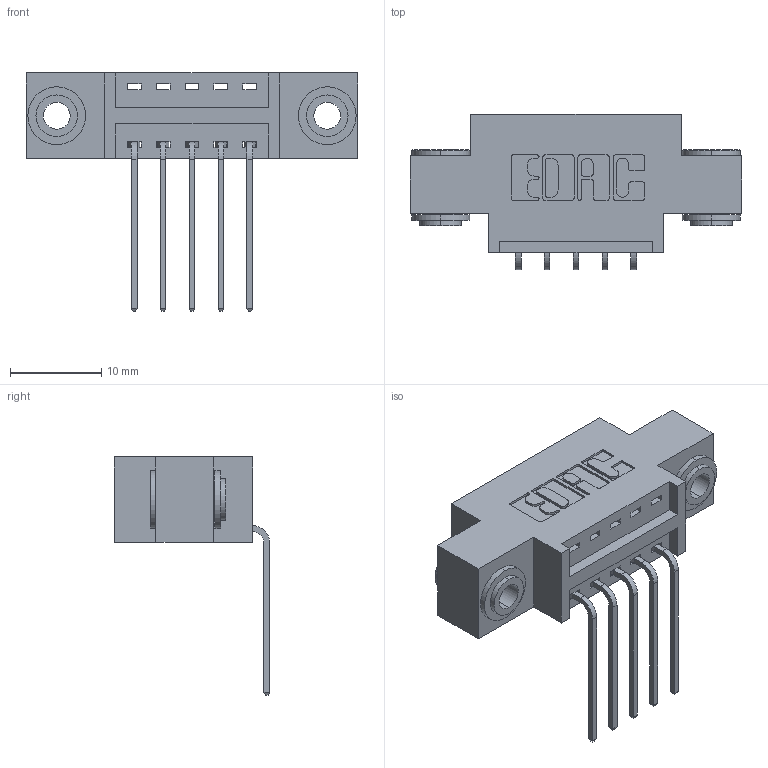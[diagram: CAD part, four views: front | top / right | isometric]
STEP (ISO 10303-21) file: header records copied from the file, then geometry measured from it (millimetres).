
FILE_DESCRIPTION (( 'STEP AP203' ), '1' );
FILE_NAME ('346-005-559-603.STEP', '2022-05-04T18:11:07', ( '' ), ( '' ), 'SwSTEP 2.0', 'SolidWorks 2020', '' );
FILE_SCHEMA (( 'CONFIG_CONTROL_DESIGN' ));
Length unit declared in the file: inch
Products named in the file (4): 346 Part_0.170 Offset - 0.156 Dia-TH; 345-250-002_345-250-002-102; 346-005-559-603; 345-292-001_558 559 Tail - 1
Assembly tree (8 placements, depth 2):
  346-005-559-603
    346 Part_0.170 Offset - 0.156 Dia-TH
    345-292-001_558 559 Tail - 1  x5
    345-250-002_345-250-002-102  x2
Bounding box: 36.45 x 17.08 x 26.16 mm (x, y, z)
Volume: 3097.4 mm3; surface area: 3983.3 mm2
Topology: 8 solids, 8 shells, 478 faces, 1363 edges, 898 vertices
Faces by surface type: plane 314, cylinder 156, cone 8
Entity records: 9366 total; most frequent: CARTESIAN_POINT 1600, ORIENTED_EDGE 1530, DIRECTION 1485, EDGE_CURVE 765, LINE 589, VECTOR 589, VERTEX_POINT 506, AXIS2_PLACEMENT_3D 448
